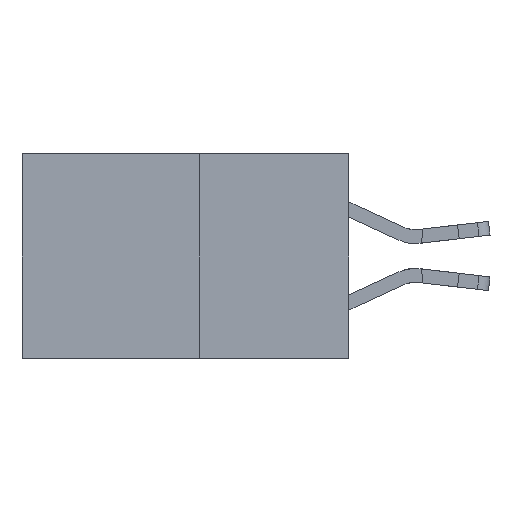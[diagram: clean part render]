
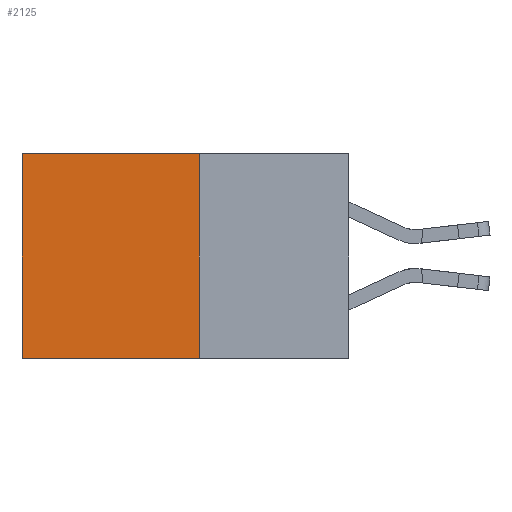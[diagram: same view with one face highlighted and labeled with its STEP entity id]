
A CAD part, left-side view. The second image highlights one B-rep face of the part: STEP entity #2125.
In plain terms, the highlighted planar face has unit normal (-1, 0, 0).
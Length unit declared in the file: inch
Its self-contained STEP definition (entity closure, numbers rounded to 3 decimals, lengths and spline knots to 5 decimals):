
#903 = VECTOR ( 'NONE', #15833, 39.37008 ) ;
#1603 = PLANE ( 'NONE',  #24040 ) ;
#1604 = VERTEX_POINT ( 'NONE', #24770 ) ;
#2125 = ADVANCED_FACE ( 'NONE', ( #10848 ), #1603, .F. ) ;
#2212 = ORIENTED_EDGE ( 'NONE', *, *, #2943, .T. ) ;
#2761 = VECTOR ( 'NONE', #9034, 39.37008 ) ;
#2943 = EDGE_CURVE ( 'NONE', #27185, #1604, #12809, .T. ) ;
#3309 = DIRECTION ( 'NONE',  ( 0., 1., 0. ) ) ;
#3469 = CARTESIAN_POINT ( 'NONE',  ( 0.277, 0.27, 0. ) ) ;
#5845 = VECTOR ( 'NONE', #3309, 39.37008 ) ;
#6236 = EDGE_CURVE ( 'NONE', #7538, #27185, #25167, .T. ) ;
#7421 = CARTESIAN_POINT ( 'NONE',  ( 0.277, 0.59, -0.37 ) ) ;
#7538 = VERTEX_POINT ( 'NONE', #3469 ) ;
#7786 = VERTEX_POINT ( 'NONE', #25469 ) ;
#8974 = CARTESIAN_POINT ( 'NONE',  ( 0.277, 0.27, 0. ) ) ;
#9034 = DIRECTION ( 'NONE',  ( 0., 1., 0. ) ) ;
#9987 = EDGE_LOOP ( 'NONE', ( #2212, #14525, #26374, #26704 ) ) ;
#10848 = FACE_OUTER_BOUND ( 'NONE', #9987, .T. ) ;
#11485 = LINE ( 'NONE', #11697, #5845 ) ;
#11553 = DIRECTION ( 'NONE',  ( 0., 0., -1. ) ) ;
#11697 = CARTESIAN_POINT ( 'NONE',  ( 0.277, 0.27, -0.37 ) ) ;
#12809 = LINE ( 'NONE', #7421, #903 ) ;
#14525 = ORIENTED_EDGE ( 'NONE', *, *, #24593, .F. ) ;
#14698 = CARTESIAN_POINT ( 'NONE',  ( 0.277, 0.27, -0.37 ) ) ;
#14959 = VECTOR ( 'NONE', #11553, 39.37008 ) ;
#15048 = DIRECTION ( 'NONE',  ( 1., 0., 0. ) ) ;
#15833 = DIRECTION ( 'NONE',  ( 0., 0., -1. ) ) ;
#16047 = DIRECTION ( 'NONE',  ( 0., 0., -1. ) ) ;
#16281 = LINE ( 'NONE', #17972, #14959 ) ;
#17972 = CARTESIAN_POINT ( 'NONE',  ( 0.277, 0.27, -0.37 ) ) ;
#21029 = CARTESIAN_POINT ( 'NONE',  ( 0.277, 0.59, 0. ) ) ;
#21813 = EDGE_CURVE ( 'NONE', #7538, #7786, #16281, .T. ) ;
#24040 = AXIS2_PLACEMENT_3D ( 'NONE', #14698, #15048, #16047 ) ;
#24593 = EDGE_CURVE ( 'NONE', #7786, #1604, #11485, .T. ) ;
#24770 = CARTESIAN_POINT ( 'NONE',  ( 0.277, 0.59, -0.37 ) ) ;
#25167 = LINE ( 'NONE', #8974, #2761 ) ;
#25469 = CARTESIAN_POINT ( 'NONE',  ( 0.277, 0.27, -0.37 ) ) ;
#26374 = ORIENTED_EDGE ( 'NONE', *, *, #21813, .F. ) ;
#26704 = ORIENTED_EDGE ( 'NONE', *, *, #6236, .T. ) ;
#27185 = VERTEX_POINT ( 'NONE', #21029 ) ;
